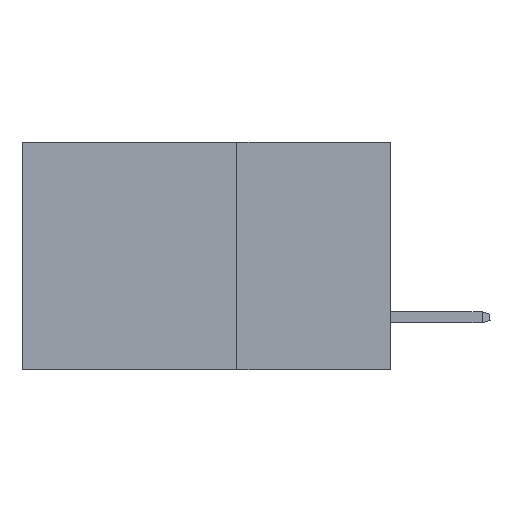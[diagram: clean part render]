
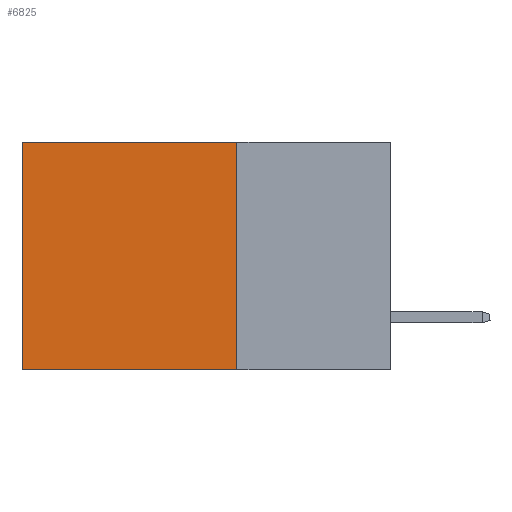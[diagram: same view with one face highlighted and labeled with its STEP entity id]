
A CAD part, left-side view. The second image highlights one B-rep face of the part: STEP entity #6825.
In plain terms, the highlighted planar face has unit normal (-1, 0, 0).
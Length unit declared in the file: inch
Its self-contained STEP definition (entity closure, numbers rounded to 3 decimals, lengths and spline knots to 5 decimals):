
#28 = EDGE_LOOP ( 'NONE', ( #4368, #18404, #18549, #6558 ) ) ;
#427 = VECTOR ( 'NONE', #12475, 39.37008 ) ;
#1825 = LINE ( 'NONE', #26908, #12774 ) ;
#1858 = CARTESIAN_POINT ( 'NONE',  ( 0.2875, 0.25, 0. ) ) ;
#2514 = DIRECTION ( 'NONE',  ( 0., 0., -1. ) ) ;
#2874 = EDGE_CURVE ( 'NONE', #20094, #12810, #15769, .T. ) ;
#3008 = CARTESIAN_POINT ( 'NONE',  ( 0.2875, 0.6, 0. ) ) ;
#3089 = CARTESIAN_POINT ( 'NONE',  ( 0.2875, 0.25, -0.37 ) ) ;
#4076 = DIRECTION ( 'NONE',  ( 0., 0., -1. ) ) ;
#4166 = VERTEX_POINT ( 'NONE', #12314 ) ;
#4368 = ORIENTED_EDGE ( 'NONE', *, *, #16620, .T. ) ;
#6558 = ORIENTED_EDGE ( 'NONE', *, *, #19493, .T. ) ;
#6825 = ADVANCED_FACE ( 'NONE', ( #27804 ), #25452, .F. ) ;
#9366 = VECTOR ( 'NONE', #18096, 39.37008 ) ;
#9446 = AXIS2_PLACEMENT_3D ( 'NONE', #1858, #17026, #4076 ) ;
#10276 = CARTESIAN_POINT ( 'NONE',  ( 0.2875, 0.6, -0.37 ) ) ;
#12314 = CARTESIAN_POINT ( 'NONE',  ( 0.2875, 0.6, 0. ) ) ;
#12448 = CARTESIAN_POINT ( 'NONE',  ( 0.2875, 0.25, -0.37 ) ) ;
#12475 = DIRECTION ( 'NONE',  ( 0., 1., 0. ) ) ;
#12774 = VECTOR ( 'NONE', #14147, 39.37008 ) ;
#12810 = VERTEX_POINT ( 'NONE', #10276 ) ;
#14147 = DIRECTION ( 'NONE',  ( 0., 1., 0. ) ) ;
#15769 = LINE ( 'NONE', #12448, #427 ) ;
#16050 = VECTOR ( 'NONE', #2514, 39.37008 ) ;
#16620 = EDGE_CURVE ( 'NONE', #4166, #12810, #21675, .T. ) ;
#17026 = DIRECTION ( 'NONE',  ( 1., 0., 0. ) ) ;
#18096 = DIRECTION ( 'NONE',  ( 0., 0., -1. ) ) ;
#18404 = ORIENTED_EDGE ( 'NONE', *, *, #2874, .F. ) ;
#18549 = ORIENTED_EDGE ( 'NONE', *, *, #20054, .F. ) ;
#19493 = EDGE_CURVE ( 'NONE', #23525, #4166, #1825, .T. ) ;
#20054 = EDGE_CURVE ( 'NONE', #23525, #20094, #22067, .T. ) ;
#20094 = VERTEX_POINT ( 'NONE', #3089 ) ;
#21675 = LINE ( 'NONE', #3008, #16050 ) ;
#22067 = LINE ( 'NONE', #26603, #9366 ) ;
#23525 = VERTEX_POINT ( 'NONE', #26221 ) ;
#25452 = PLANE ( 'NONE',  #9446 ) ;
#26221 = CARTESIAN_POINT ( 'NONE',  ( 0.2875, 0.25, 0. ) ) ;
#26603 = CARTESIAN_POINT ( 'NONE',  ( 0.2875, 0.25, 0. ) ) ;
#26908 = CARTESIAN_POINT ( 'NONE',  ( 0.2875, 0.25, 0. ) ) ;
#27804 = FACE_OUTER_BOUND ( 'NONE', #28, .T. ) ;
